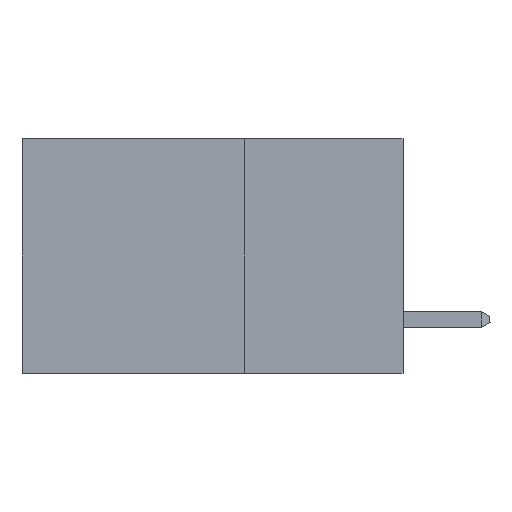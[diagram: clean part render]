
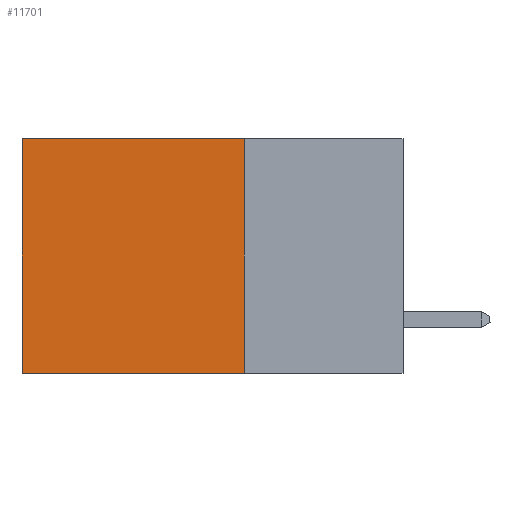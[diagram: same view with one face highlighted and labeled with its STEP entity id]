
A CAD part, left-side view. The second image highlights one B-rep face of the part: STEP entity #11701.
In plain terms, the highlighted planar face has unit normal (-1, 0, 0).
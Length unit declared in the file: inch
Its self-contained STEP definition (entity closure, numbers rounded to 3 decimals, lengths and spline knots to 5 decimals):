
#664 = EDGE_CURVE ( 'NONE', #8106, #9435, #19132, .T. ) ;
#854 = CARTESIAN_POINT ( 'NONE',  ( 0.2875, 0.25, -0.37 ) ) ;
#1474 = PLANE ( 'NONE',  #10846 ) ;
#2259 = LINE ( 'NONE', #23536, #3377 ) ;
#2386 = ORIENTED_EDGE ( 'NONE', *, *, #664, .F. ) ;
#3350 = ORIENTED_EDGE ( 'NONE', *, *, #10359, .T. ) ;
#3377 = VECTOR ( 'NONE', #19033, 39.37008 ) ;
#4892 = VERTEX_POINT ( 'NONE', #21363 ) ;
#5113 = DIRECTION ( 'NONE',  ( 0., 0., -1. ) ) ;
#6158 = CARTESIAN_POINT ( 'NONE',  ( 0.2875, 0.25, 0. ) ) ;
#6214 = DIRECTION ( 'NONE',  ( 0., 1., 0. ) ) ;
#7210 = VECTOR ( 'NONE', #5113, 39.37008 ) ;
#7674 = CARTESIAN_POINT ( 'NONE',  ( 0.2875, 0.6, 0. ) ) ;
#8106 = VERTEX_POINT ( 'NONE', #6158 ) ;
#8687 = EDGE_CURVE ( 'NONE', #12071, #4892, #2259, .T. ) ;
#8920 = CARTESIAN_POINT ( 'NONE',  ( 0.2875, 0.25, 0. ) ) ;
#9412 = CARTESIAN_POINT ( 'NONE',  ( 0.2875, 0.25, 0. ) ) ;
#9435 = VERTEX_POINT ( 'NONE', #14699 ) ;
#10359 = EDGE_CURVE ( 'NONE', #8106, #12071, #12198, .T. ) ;
#10663 = DIRECTION ( 'NONE',  ( 1., 0., 0. ) ) ;
#10846 = AXIS2_PLACEMENT_3D ( 'NONE', #8920, #10663, #23326 ) ;
#11701 = ADVANCED_FACE ( 'NONE', ( #23212 ), #1474, .F. ) ;
#12071 = VERTEX_POINT ( 'NONE', #7674 ) ;
#12198 = LINE ( 'NONE', #9412, #21554 ) ;
#12484 = DIRECTION ( 'NONE',  ( 0., 1., 0. ) ) ;
#14699 = CARTESIAN_POINT ( 'NONE',  ( 0.2875, 0.25, -0.37 ) ) ;
#15254 = VECTOR ( 'NONE', #6214, 39.37008 ) ;
#16971 = LINE ( 'NONE', #854, #15254 ) ;
#19033 = DIRECTION ( 'NONE',  ( 0., 0., -1. ) ) ;
#19132 = LINE ( 'NONE', #21575, #7210 ) ;
#20797 = ORIENTED_EDGE ( 'NONE', *, *, #22912, .F. ) ;
#21363 = CARTESIAN_POINT ( 'NONE',  ( 0.2875, 0.6, -0.37 ) ) ;
#21554 = VECTOR ( 'NONE', #12484, 39.37008 ) ;
#21575 = CARTESIAN_POINT ( 'NONE',  ( 0.2875, 0.25, 0. ) ) ;
#22417 = ORIENTED_EDGE ( 'NONE', *, *, #8687, .T. ) ;
#22912 = EDGE_CURVE ( 'NONE', #9435, #4892, #16971, .T. ) ;
#23020 = EDGE_LOOP ( 'NONE', ( #22417, #20797, #2386, #3350 ) ) ;
#23212 = FACE_OUTER_BOUND ( 'NONE', #23020, .T. ) ;
#23326 = DIRECTION ( 'NONE',  ( 0., 0., -1. ) ) ;
#23536 = CARTESIAN_POINT ( 'NONE',  ( 0.2875, 0.6, 0. ) ) ;
